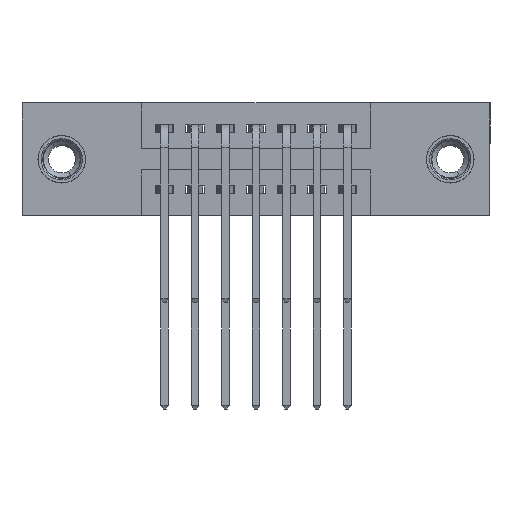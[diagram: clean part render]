
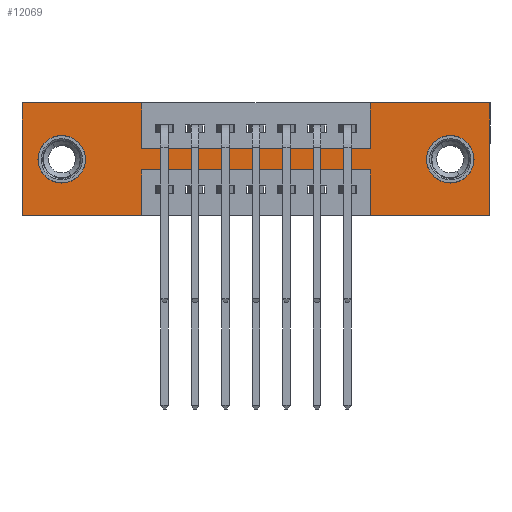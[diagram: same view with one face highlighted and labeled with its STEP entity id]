
A CAD part, front view. The second image highlights one B-rep face of the part: STEP entity #12069.
In plain terms, the highlighted planar face has unit normal (0, -1, 0).
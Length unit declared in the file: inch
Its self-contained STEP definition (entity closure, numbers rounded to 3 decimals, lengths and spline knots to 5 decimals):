
#253 = CARTESIAN_POINT ( 'NONE',  ( 1.405, 0., -0.185 ) ) ;
#421 = CARTESIAN_POINT ( 'NONE',  ( 0., 0., -0.37 ) ) ;
#655 = VECTOR ( 'NONE', #15175, 39.37008 ) ;
#675 = VERTEX_POINT ( 'NONE', #10443 ) ;
#733 = AXIS2_PLACEMENT_3D ( 'NONE', #11636, #2481, #2533 ) ;
#825 = CARTESIAN_POINT ( 'NONE',  ( 0.3925, 0., -0.15 ) ) ;
#1073 = CARTESIAN_POINT ( 'NONE',  ( 1.405, 0., -0.185 ) ) ;
#1217 = VERTEX_POINT ( 'NONE', #6959 ) ;
#1755 = VERTEX_POINT ( 'NONE', #4528 ) ;
#1884 = VECTOR ( 'NONE', #5226, 39.37008 ) ;
#2000 = AXIS2_PLACEMENT_3D ( 'NONE', #1073, #9965, #2306 ) ;
#2073 = CIRCLE ( 'NONE', #2000, 0.078 ) ;
#2212 = ORIENTED_EDGE ( 'NONE', *, *, #9105, .F. ) ;
#2306 = DIRECTION ( 'NONE',  ( 0., 0., -1. ) ) ;
#2398 = VERTEX_POINT ( 'NONE', #7514 ) ;
#2425 = CARTESIAN_POINT ( 'NONE',  ( 0., 0., -0.37 ) ) ;
#2481 = DIRECTION ( 'NONE',  ( 0., -1., 0. ) ) ;
#2533 = DIRECTION ( 'NONE',  ( 0., 0., -1. ) ) ;
#2639 = DIRECTION ( 'NONE',  ( -1., 0., 0. ) ) ;
#2757 = CARTESIAN_POINT ( 'NONE',  ( 0.13, 0., -0.185 ) ) ;
#2758 = FACE_BOUND ( 'NONE', #14744, .T. ) ;
#2864 = VECTOR ( 'NONE', #4007, 39.37008 ) ;
#2869 = CARTESIAN_POINT ( 'NONE',  ( 1.1425, 0., -0.37 ) ) ;
#2888 = CARTESIAN_POINT ( 'NONE',  ( 1.1425, 0., 0. ) ) ;
#2953 = CARTESIAN_POINT ( 'NONE',  ( 1.405, 0., -0.107 ) ) ;
#3022 = CARTESIAN_POINT ( 'NONE',  ( 1.405, 0., -0.263 ) ) ;
#3223 = VECTOR ( 'NONE', #13668, 39.37008 ) ;
#3342 = CARTESIAN_POINT ( 'NONE',  ( 0., 0., 0. ) ) ;
#3370 = VERTEX_POINT ( 'NONE', #4558 ) ;
#3478 = EDGE_CURVE ( 'NONE', #11145, #5264, #2073, .T. ) ;
#3728 = LINE ( 'NONE', #2869, #11006 ) ;
#3850 = VECTOR ( 'NONE', #10962, 39.37008 ) ;
#3876 = AXIS2_PLACEMENT_3D ( 'NONE', #2757, #5392, #11751 ) ;
#3955 = EDGE_CURVE ( 'NONE', #675, #15160, #14283, .T. ) ;
#4007 = DIRECTION ( 'NONE',  ( -1., 0., 0. ) ) ;
#4009 = DIRECTION ( 'NONE',  ( 0., 0., -1. ) ) ;
#4173 = VECTOR ( 'NONE', #5527, 39.37008 ) ;
#4229 = VERTEX_POINT ( 'NONE', #12161 ) ;
#4305 = CARTESIAN_POINT ( 'NONE',  ( 0.13, 0., -0.185 ) ) ;
#4383 = VECTOR ( 'NONE', #12353, 39.37008 ) ;
#4408 = ORIENTED_EDGE ( 'NONE', *, *, #6131, .F. ) ;
#4528 = CARTESIAN_POINT ( 'NONE',  ( 0.13, 0., -0.263 ) ) ;
#4558 = CARTESIAN_POINT ( 'NONE',  ( 0.3925, 0., -0.22 ) ) ;
#4578 = EDGE_CURVE ( 'NONE', #15160, #16191, #8996, .T. ) ;
#4771 = CARTESIAN_POINT ( 'NONE',  ( 0.3925, 0., -0.37 ) ) ;
#4837 = EDGE_CURVE ( 'NONE', #16191, #5459, #9401, .T. ) ;
#5070 = DIRECTION ( 'NONE',  ( 0., 0., 1. ) ) ;
#5165 = AXIS2_PLACEMENT_3D ( 'NONE', #4305, #10797, #12262 ) ;
#5226 = DIRECTION ( 'NONE',  ( 0., 0., -1. ) ) ;
#5264 = VERTEX_POINT ( 'NONE', #3022 ) ;
#5388 = VECTOR ( 'NONE', #2639, 39.37008 ) ;
#5392 = DIRECTION ( 'NONE',  ( 0., 1., 0. ) ) ;
#5459 = VERTEX_POINT ( 'NONE', #9120 ) ;
#5527 = DIRECTION ( 'NONE',  ( 0., 0., 1. ) ) ;
#5608 = LINE ( 'NONE', #13854, #655 ) ;
#5663 = VERTEX_POINT ( 'NONE', #16385 ) ;
#5730 = CIRCLE ( 'NONE', #5165, 0.078 ) ;
#5792 = EDGE_CURVE ( 'NONE', #1755, #6386, #5730, .T. ) ;
#5876 = VERTEX_POINT ( 'NONE', #7714 ) ;
#6011 = ORIENTED_EDGE ( 'NONE', *, *, #15837, .T. ) ;
#6131 = EDGE_CURVE ( 'NONE', #9010, #2398, #3728, .T. ) ;
#6241 = LINE ( 'NONE', #12964, #1884 ) ;
#6386 = VERTEX_POINT ( 'NONE', #14708 ) ;
#6614 = CIRCLE ( 'NONE', #3876, 0.078 ) ;
#6751 = ORIENTED_EDGE ( 'NONE', *, *, #9223, .F. ) ;
#6959 = CARTESIAN_POINT ( 'NONE',  ( 0., 0., 0. ) ) ;
#7041 = EDGE_CURVE ( 'NONE', #2398, #3370, #16250, .T. ) ;
#7058 = VECTOR ( 'NONE', #5070, 39.37008 ) ;
#7077 = ORIENTED_EDGE ( 'NONE', *, *, #13984, .F. ) ;
#7144 = ORIENTED_EDGE ( 'NONE', *, *, #7041, .F. ) ;
#7232 = DIRECTION ( 'NONE',  ( 0., 0., 1. ) ) ;
#7514 = CARTESIAN_POINT ( 'NONE',  ( 1.1425, 0., -0.22 ) ) ;
#7549 = ORIENTED_EDGE ( 'NONE', *, *, #9351, .F. ) ;
#7714 = CARTESIAN_POINT ( 'NONE',  ( 0.3925, 0., 0. ) ) ;
#7879 = DIRECTION ( 'NONE',  ( 0., 1., 0. ) ) ;
#8694 = EDGE_CURVE ( 'NONE', #3370, #5663, #14529, .T. ) ;
#8800 = EDGE_CURVE ( 'NONE', #6386, #1755, #6614, .T. ) ;
#8832 = CARTESIAN_POINT ( 'NONE',  ( 1.1425, 0., 0. ) ) ;
#8996 = LINE ( 'NONE', #2888, #4173 ) ;
#9010 = VERTEX_POINT ( 'NONE', #12955 ) ;
#9105 = EDGE_CURVE ( 'NONE', #5663, #10834, #10481, .T. ) ;
#9120 = CARTESIAN_POINT ( 'NONE',  ( 1.535, 0., 0. ) ) ;
#9223 = EDGE_CURVE ( 'NONE', #4229, #9010, #15324, .T. ) ;
#9351 = EDGE_CURVE ( 'NONE', #5876, #675, #5608, .T. ) ;
#9401 = LINE ( 'NONE', #3342, #4383 ) ;
#9462 = ORIENTED_EDGE ( 'NONE', *, *, #4578, .F. ) ;
#9965 = DIRECTION ( 'NONE',  ( 0., 1., 0. ) ) ;
#9986 = FACE_BOUND ( 'NONE', #12750, .T. ) ;
#10443 = CARTESIAN_POINT ( 'NONE',  ( 0.3925, 0., -0.15 ) ) ;
#10481 = LINE ( 'NONE', #421, #2864 ) ;
#10727 = LINE ( 'NONE', #13702, #3850 ) ;
#10797 = DIRECTION ( 'NONE',  ( 0., 1., 0. ) ) ;
#10834 = VERTEX_POINT ( 'NONE', #15994 ) ;
#10962 = DIRECTION ( 'NONE',  ( 1., 0., 0. ) ) ;
#11006 = VECTOR ( 'NONE', #7232, 39.37008 ) ;
#11145 = VERTEX_POINT ( 'NONE', #2953 ) ;
#11250 = EDGE_LOOP ( 'NONE', ( #16485, #7144, #4408, #6751, #7077, #14952, #9462, #13709, #7549, #15090, #14701, #2212 ) ) ;
#11312 = CARTESIAN_POINT ( 'NONE',  ( 0.3925, 0., -0.22 ) ) ;
#11422 = DIRECTION ( 'NONE',  ( -1., 0., 0. ) ) ;
#11636 = CARTESIAN_POINT ( 'NONE',  ( 0., 0., -0.37 ) ) ;
#11751 = DIRECTION ( 'NONE',  ( 0., 0., 1. ) ) ;
#12069 = ADVANCED_FACE ( 'NONE', ( #9986, #2758, #15241 ), #14151, .T. ) ;
#12161 = CARTESIAN_POINT ( 'NONE',  ( 1.535, 0., -0.37 ) ) ;
#12262 = DIRECTION ( 'NONE',  ( 0., 0., 1. ) ) ;
#12353 = DIRECTION ( 'NONE',  ( 1., 0., 0. ) ) ;
#12742 = ORIENTED_EDGE ( 'NONE', *, *, #3478, .T. ) ;
#12750 = EDGE_LOOP ( 'NONE', ( #12742, #6011 ) ) ;
#12955 = CARTESIAN_POINT ( 'NONE',  ( 1.1425, 0., -0.37 ) ) ;
#12964 = CARTESIAN_POINT ( 'NONE',  ( 1.535, 0., 0. ) ) ;
#12980 = CARTESIAN_POINT ( 'NONE',  ( 1.1425, 0., -0.15 ) ) ;
#13668 = DIRECTION ( 'NONE',  ( 1., 0., 0. ) ) ;
#13702 = CARTESIAN_POINT ( 'NONE',  ( 0., 0., 0. ) ) ;
#13709 = ORIENTED_EDGE ( 'NONE', *, *, #3955, .F. ) ;
#13809 = VECTOR ( 'NONE', #11422, 39.37008 ) ;
#13854 = CARTESIAN_POINT ( 'NONE',  ( 0.3925, 0., 0. ) ) ;
#13984 = EDGE_CURVE ( 'NONE', #5459, #4229, #6241, .T. ) ;
#14151 = PLANE ( 'NONE',  #733 ) ;
#14178 = ORIENTED_EDGE ( 'NONE', *, *, #5792, .T. ) ;
#14223 = EDGE_CURVE ( 'NONE', #1217, #5876, #10727, .T. ) ;
#14283 = LINE ( 'NONE', #825, #3223 ) ;
#14342 = LINE ( 'NONE', #15386, #7058 ) ;
#14529 = LINE ( 'NONE', #4771, #16158 ) ;
#14701 = ORIENTED_EDGE ( 'NONE', *, *, #15215, .F. ) ;
#14708 = CARTESIAN_POINT ( 'NONE',  ( 0.13, 0., -0.107 ) ) ;
#14744 = EDGE_LOOP ( 'NONE', ( #16506, #14178 ) ) ;
#14952 = ORIENTED_EDGE ( 'NONE', *, *, #4837, .F. ) ;
#15082 = AXIS2_PLACEMENT_3D ( 'NONE', #253, #7879, #4009 ) ;
#15090 = ORIENTED_EDGE ( 'NONE', *, *, #14223, .F. ) ;
#15104 = DIRECTION ( 'NONE',  ( 0., 0., -1. ) ) ;
#15160 = VERTEX_POINT ( 'NONE', #12980 ) ;
#15175 = DIRECTION ( 'NONE',  ( 0., 0., -1. ) ) ;
#15215 = EDGE_CURVE ( 'NONE', #10834, #1217, #14342, .T. ) ;
#15241 = FACE_OUTER_BOUND ( 'NONE', #11250, .T. ) ;
#15324 = LINE ( 'NONE', #2425, #5388 ) ;
#15386 = CARTESIAN_POINT ( 'NONE',  ( 0., 0., 0. ) ) ;
#15837 = EDGE_CURVE ( 'NONE', #5264, #11145, #16442, .T. ) ;
#15994 = CARTESIAN_POINT ( 'NONE',  ( 0., 0., -0.37 ) ) ;
#16158 = VECTOR ( 'NONE', #15104, 39.37008 ) ;
#16191 = VERTEX_POINT ( 'NONE', #8832 ) ;
#16250 = LINE ( 'NONE', #11312, #13809 ) ;
#16385 = CARTESIAN_POINT ( 'NONE',  ( 0.3925, 0., -0.37 ) ) ;
#16442 = CIRCLE ( 'NONE', #15082, 0.078 ) ;
#16485 = ORIENTED_EDGE ( 'NONE', *, *, #8694, .F. ) ;
#16506 = ORIENTED_EDGE ( 'NONE', *, *, #8800, .T. ) ;
